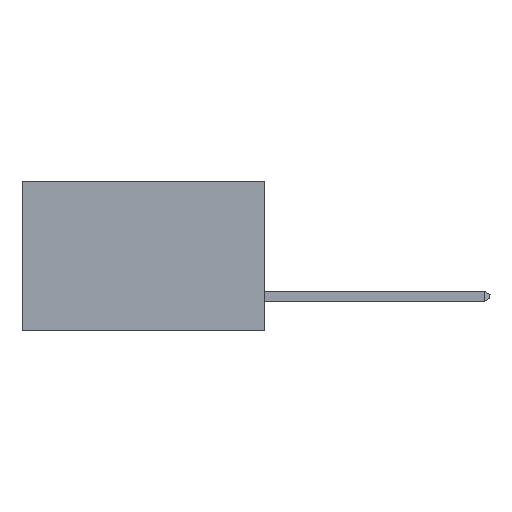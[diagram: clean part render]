
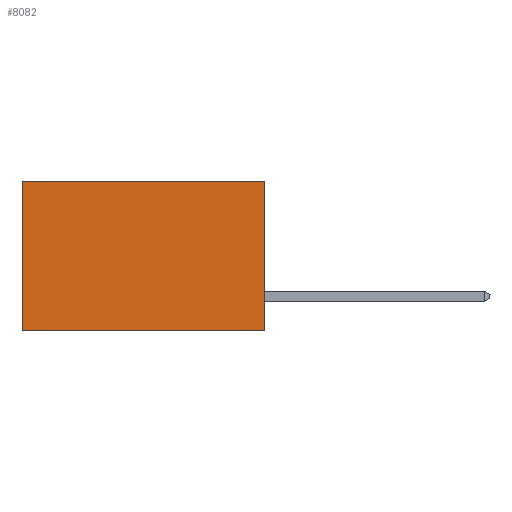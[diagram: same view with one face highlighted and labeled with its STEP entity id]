
A CAD part, left-side view. The second image highlights one B-rep face of the part: STEP entity #8082.
In plain terms, the highlighted planar face has unit normal (-1, 0, 0).
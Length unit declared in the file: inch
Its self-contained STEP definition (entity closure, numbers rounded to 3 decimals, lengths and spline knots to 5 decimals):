
#3 = CARTESIAN_POINT ( 'NONE',  ( 0.2615, 0., -0.37 ) ) ;
#92 = CARTESIAN_POINT ( 'NONE',  ( 0.2615, 0.6, 0. ) ) ;
#908 = DIRECTION ( 'NONE',  ( 1., 0., 0. ) ) ;
#1599 = EDGE_LOOP ( 'NONE', ( #2254, #15429, #9158, #18453 ) ) ;
#2254 = ORIENTED_EDGE ( 'NONE', *, *, #3701, .T. ) ;
#3366 = EDGE_CURVE ( 'NONE', #4987, #23633, #13091, .T. ) ;
#3701 = EDGE_CURVE ( 'NONE', #21301, #21961, #15374, .T. ) ;
#4669 = EDGE_CURVE ( 'NONE', #23633, #21961, #17316, .T. ) ;
#4987 = VERTEX_POINT ( 'NONE', #11323 ) ;
#5383 = DIRECTION ( 'NONE',  ( 0., 0., -1. ) ) ;
#6224 = FACE_OUTER_BOUND ( 'NONE', #1599, .T. ) ;
#6987 = CARTESIAN_POINT ( 'NONE',  ( 0.2615, 0.6, -0.37 ) ) ;
#8082 = ADVANCED_FACE ( 'NONE', ( #6224 ), #19743, .F. ) ;
#8477 = CARTESIAN_POINT ( 'NONE',  ( 0.2615, 0., -0.37 ) ) ;
#9158 = ORIENTED_EDGE ( 'NONE', *, *, #3366, .F. ) ;
#10480 = CARTESIAN_POINT ( 'NONE',  ( 0.2615, 0., 0. ) ) ;
#10607 = LINE ( 'NONE', #10480, #13915 ) ;
#11322 = DIRECTION ( 'NONE',  ( 0., 0., -1. ) ) ;
#11323 = CARTESIAN_POINT ( 'NONE',  ( 0.2615, 0., 0. ) ) ;
#11798 = VECTOR ( 'NONE', #5383, 39.37008 ) ;
#12045 = EDGE_CURVE ( 'NONE', #4987, #21301, #10607, .T. ) ;
#13091 = LINE ( 'NONE', #20805, #23907 ) ;
#13504 = DIRECTION ( 'NONE',  ( 0., 1., 0. ) ) ;
#13915 = VECTOR ( 'NONE', #16292, 39.37008 ) ;
#15374 = LINE ( 'NONE', #20799, #11798 ) ;
#15429 = ORIENTED_EDGE ( 'NONE', *, *, #4669, .F. ) ;
#15514 = VECTOR ( 'NONE', #13504, 39.37008 ) ;
#16292 = DIRECTION ( 'NONE',  ( 0., 1., 0. ) ) ;
#17316 = LINE ( 'NONE', #3, #15514 ) ;
#18453 = ORIENTED_EDGE ( 'NONE', *, *, #12045, .T. ) ;
#19743 = PLANE ( 'NONE',  #20912 ) ;
#20799 = CARTESIAN_POINT ( 'NONE',  ( 0.2615, 0.6, -0.37 ) ) ;
#20805 = CARTESIAN_POINT ( 'NONE',  ( 0.2615, 0., -0.37 ) ) ;
#20912 = AXIS2_PLACEMENT_3D ( 'NONE', #8477, #908, #22012 ) ;
#21301 = VERTEX_POINT ( 'NONE', #92 ) ;
#21961 = VERTEX_POINT ( 'NONE', #6987 ) ;
#22012 = DIRECTION ( 'NONE',  ( 0., 0., -1. ) ) ;
#23633 = VERTEX_POINT ( 'NONE', #24136 ) ;
#23907 = VECTOR ( 'NONE', #11322, 39.37008 ) ;
#24136 = CARTESIAN_POINT ( 'NONE',  ( 0.2615, 0., -0.37 ) ) ;
